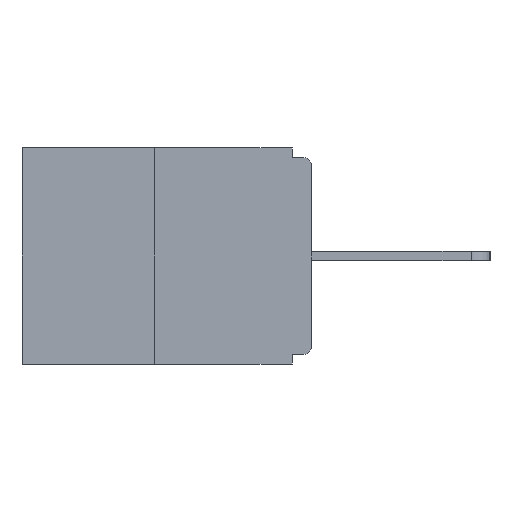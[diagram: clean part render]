
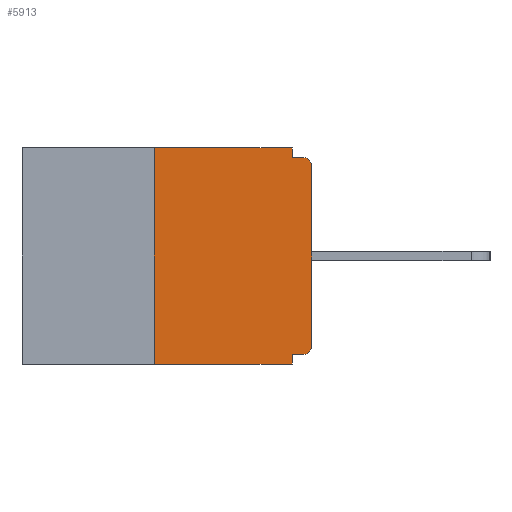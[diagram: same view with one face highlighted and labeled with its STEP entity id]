
A CAD part, left-side view. The second image highlights one B-rep face of the part: STEP entity #5913.
In plain terms, the highlighted planar face has unit normal (-1, 0, 0).
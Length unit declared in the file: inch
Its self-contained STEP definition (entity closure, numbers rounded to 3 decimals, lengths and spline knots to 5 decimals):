
#72 = PLANE ( 'NONE',  #804 ) ;
#627 = VECTOR ( 'NONE', #19741, 39.37008 ) ;
#804 = AXIS2_PLACEMENT_3D ( 'NONE', #8674, #1564, #1509 ) ;
#899 = CARTESIAN_POINT ( 'NONE',  ( 0., 0.031, -0.343 ) ) ;
#922 = VERTEX_POINT ( 'NONE', #899 ) ;
#1509 = DIRECTION ( 'NONE',  ( 0., 0., -1. ) ) ;
#1564 = DIRECTION ( 'NONE',  ( 1., 0., 0. ) ) ;
#1615 = CARTESIAN_POINT ( 'NONE',  ( 0., 0.015, -0.313 ) ) ;
#1619 = VECTOR ( 'NONE', #18935, 39.37008 ) ;
#1739 = VECTOR ( 'NONE', #21140, 39.37008 ) ;
#1907 = AXIS2_PLACEMENT_3D ( 'NONE', #1615, #14428, #3505 ) ;
#3050 = VECTOR ( 'NONE', #9037, 39.37008 ) ;
#3434 = CARTESIAN_POINT ( 'NONE',  ( 0., 0., -0.03 ) ) ;
#3505 = DIRECTION ( 'NONE',  ( 0., 0., -1. ) ) ;
#3636 = LINE ( 'NONE', #21389, #3050 ) ;
#3975 = CARTESIAN_POINT ( 'NONE',  ( 0., 0.031, -0.343 ) ) ;
#4819 = CIRCLE ( 'NONE', #1907, 0.015 ) ;
#4826 = ORIENTED_EDGE ( 'NONE', *, *, #6537, .F. ) ;
#4932 = EDGE_LOOP ( 'NONE', ( #4826, #6154, #6223, #7112, #7323, #7525, #7562, #7868, #8152, #8174 ) ) ;
#5128 = CARTESIAN_POINT ( 'NONE',  ( 0., 0., 0. ) ) ;
#5295 = VERTEX_POINT ( 'NONE', #8982 ) ;
#5303 = VECTOR ( 'NONE', #9538, 39.37008 ) ;
#5913 = ADVANCED_FACE ( 'NONE', ( #20197 ), #72, .F. ) ;
#6154 = ORIENTED_EDGE ( 'NONE', *, *, #21314, .F. ) ;
#6207 = VERTEX_POINT ( 'NONE', #15426 ) ;
#6223 = ORIENTED_EDGE ( 'NONE', *, *, #15539, .T. ) ;
#6537 = EDGE_CURVE ( 'NONE', #13681, #22998, #21488, .T. ) ;
#6979 = DIRECTION ( 'NONE',  ( 0., 0., 1. ) ) ;
#7000 = VERTEX_POINT ( 'NONE', #15296 ) ;
#7112 = ORIENTED_EDGE ( 'NONE', *, *, #20655, .F. ) ;
#7223 = CARTESIAN_POINT ( 'NONE',  ( 0., 0.46, 0. ) ) ;
#7323 = ORIENTED_EDGE ( 'NONE', *, *, #22892, .F. ) ;
#7525 = ORIENTED_EDGE ( 'NONE', *, *, #14610, .T. ) ;
#7562 = ORIENTED_EDGE ( 'NONE', *, *, #19846, .T. ) ;
#7868 = ORIENTED_EDGE ( 'NONE', *, *, #19334, .T. ) ;
#8152 = ORIENTED_EDGE ( 'NONE', *, *, #15022, .F. ) ;
#8168 = DIRECTION ( 'NONE',  ( 0., -1., 0. ) ) ;
#8174 = ORIENTED_EDGE ( 'NONE', *, *, #12140, .F. ) ;
#8198 = CARTESIAN_POINT ( 'NONE',  ( 0., 0., -0.015 ) ) ;
#8674 = CARTESIAN_POINT ( 'NONE',  ( 0., 0.46, 0. ) ) ;
#8792 = DIRECTION ( 'NONE',  ( -1., 0., 0. ) ) ;
#8982 = CARTESIAN_POINT ( 'NONE',  ( 0., 0., -0.313 ) ) ;
#9037 = DIRECTION ( 'NONE',  ( 0., -1., 0. ) ) ;
#9350 = CARTESIAN_POINT ( 'NONE',  ( 0., 0.015, -0.328 ) ) ;
#9538 = DIRECTION ( 'NONE',  ( 0., 0., -1. ) ) ;
#9679 = VECTOR ( 'NONE', #6979, 39.37008 ) ;
#9734 = VERTEX_POINT ( 'NONE', #3434 ) ;
#9803 = VERTEX_POINT ( 'NONE', #9350 ) ;
#10584 = CARTESIAN_POINT ( 'NONE',  ( 0., 0.031, 0. ) ) ;
#10655 = LINE ( 'NONE', #15920, #19519 ) ;
#10792 = LINE ( 'NONE', #3975, #5303 ) ;
#10964 = AXIS2_PLACEMENT_3D ( 'NONE', #19463, #8792, #21182 ) ;
#10970 = LINE ( 'NONE', #10584, #1739 ) ;
#12078 = VERTEX_POINT ( 'NONE', #19349 ) ;
#12140 = EDGE_CURVE ( 'NONE', #22998, #12078, #10970, .T. ) ;
#13294 = VECTOR ( 'NONE', #8168, 39.37008 ) ;
#13681 = VERTEX_POINT ( 'NONE', #16996 ) ;
#14428 = DIRECTION ( 'NONE',  ( -1., 0., 0. ) ) ;
#14489 = LINE ( 'NONE', #5128, #9679 ) ;
#14610 = EDGE_CURVE ( 'NONE', #9803, #5295, #4819, .T. ) ;
#15022 = EDGE_CURVE ( 'NONE', #12078, #15693, #19715, .T. ) ;
#15296 = CARTESIAN_POINT ( 'NONE',  ( 0., 0.031, -0.328 ) ) ;
#15426 = CARTESIAN_POINT ( 'NONE',  ( 0., 0.25, -0.343 ) ) ;
#15539 = EDGE_CURVE ( 'NONE', #6207, #922, #3636, .T. ) ;
#15693 = VERTEX_POINT ( 'NONE', #16697 ) ;
#15920 = CARTESIAN_POINT ( 'NONE',  ( 0., 0., -0.328 ) ) ;
#16393 = CIRCLE ( 'NONE', #10964, 0.015 ) ;
#16697 = CARTESIAN_POINT ( 'NONE',  ( 0., 0.015, -0.015 ) ) ;
#16996 = CARTESIAN_POINT ( 'NONE',  ( 0., 0.25, 0. ) ) ;
#18012 = CARTESIAN_POINT ( 'NONE',  ( 0., 0.25, 0. ) ) ;
#18014 = CARTESIAN_POINT ( 'NONE',  ( 0., 0.031, 0. ) ) ;
#18935 = DIRECTION ( 'NONE',  ( 0., -1., 0. ) ) ;
#19334 = EDGE_CURVE ( 'NONE', #9734, #15693, #16393, .T. ) ;
#19349 = CARTESIAN_POINT ( 'NONE',  ( 0., 0.031, -0.015 ) ) ;
#19437 = DIRECTION ( 'NONE',  ( 0., 1., 0. ) ) ;
#19463 = CARTESIAN_POINT ( 'NONE',  ( 0., 0.015, -0.03 ) ) ;
#19519 = VECTOR ( 'NONE', #19437, 39.37008 ) ;
#19715 = LINE ( 'NONE', #8198, #1619 ) ;
#19741 = DIRECTION ( 'NONE',  ( 0., 0., 1. ) ) ;
#19846 = EDGE_CURVE ( 'NONE', #5295, #9734, #14489, .T. ) ;
#19882 = LINE ( 'NONE', #18012, #627 ) ;
#20197 = FACE_OUTER_BOUND ( 'NONE', #4932, .T. ) ;
#20655 = EDGE_CURVE ( 'NONE', #7000, #922, #10792, .T. ) ;
#21140 = DIRECTION ( 'NONE',  ( 0., 0., -1. ) ) ;
#21182 = DIRECTION ( 'NONE',  ( 0., 0., -1. ) ) ;
#21314 = EDGE_CURVE ( 'NONE', #6207, #13681, #19882, .T. ) ;
#21389 = CARTESIAN_POINT ( 'NONE',  ( 0., 0.46, -0.343 ) ) ;
#21488 = LINE ( 'NONE', #7223, #13294 ) ;
#22892 = EDGE_CURVE ( 'NONE', #9803, #7000, #10655, .T. ) ;
#22998 = VERTEX_POINT ( 'NONE', #18014 ) ;
